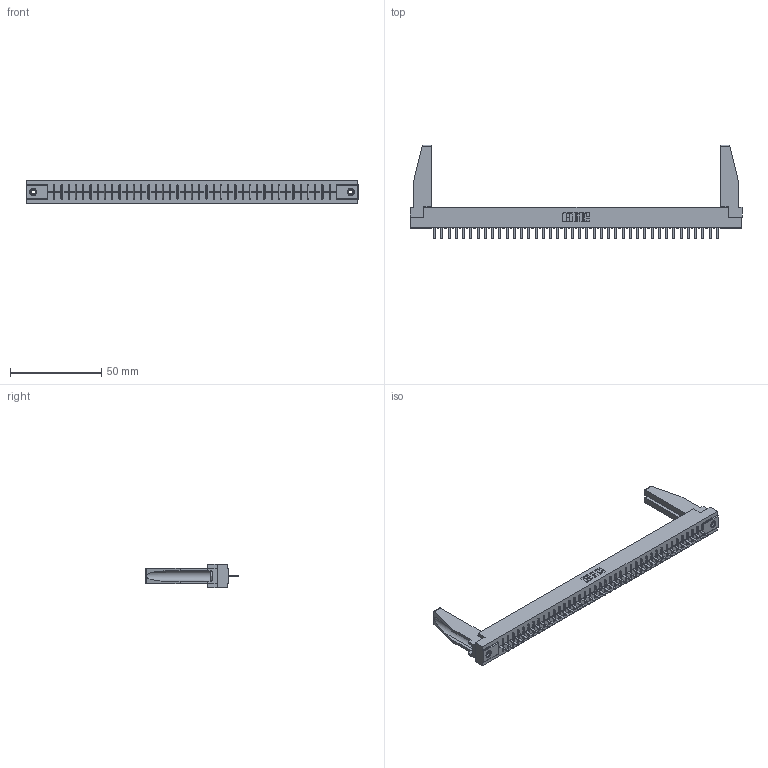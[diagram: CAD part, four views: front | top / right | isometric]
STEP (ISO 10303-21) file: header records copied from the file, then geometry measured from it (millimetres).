
FILE_DESCRIPTION (( 'STEP AP203' ), '1' );
FILE_NAME ('356-040-420-178.STEP', '2020-09-24T00:38:20', ( '' ), ( '' ), 'SwSTEP 2.0', 'SolidWorks 2020', '' );
FILE_SCHEMA (( 'CONFIG_CONTROL_DESIGN' ));
Length unit declared in the file: inch
Products named in the file (5): 307-220-078; 306-290-001_120; 356-040-420-178; 345-250-001_345-250-001-102; 306 Part_.156 Dia
Assembly tree (45 placements, depth 2):
  356-040-420-178
    306 Part_.156 Dia
    306-290-001_120  x40
    345-250-001_345-250-001-102  x2
    307-220-078  x2
Bounding box: 181.51 x 51.16 x 12.7 mm (x, y, z)
Volume: 24053.4 mm3; surface area: 24418.4 mm2
Topology: 45 solids, 45 shells, 3046 faces, 8526 edges, 5460 vertices
Faces by surface type: plane 2032, cylinder 838, sphere 160, cone 12, torus 4
Entity records: 39956 total; most frequent: CARTESIAN_POINT 6709, ORIENTED_EDGE 6610, DIRECTION 6567, EDGE_CURVE 3305, VECTOR 2587, LINE 2587, VERTEX_POINT 2090, AXIS2_PLACEMENT_3D 1990
